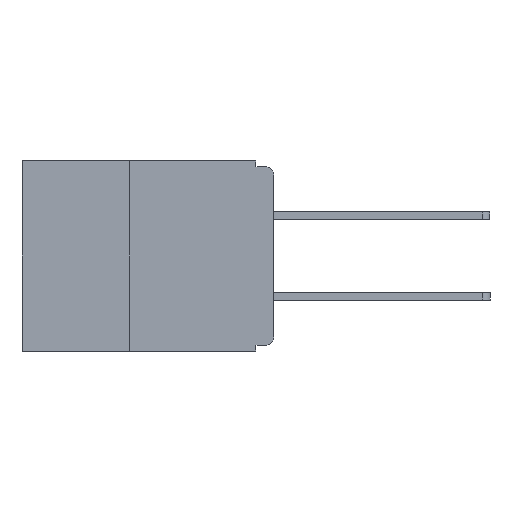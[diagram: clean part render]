
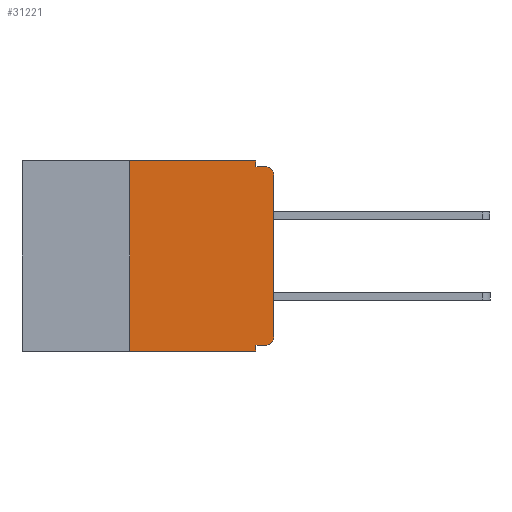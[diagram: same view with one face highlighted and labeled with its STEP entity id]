
A CAD part, left-side view. The second image highlights one B-rep face of the part: STEP entity #31221.
In plain terms, the highlighted planar face has unit normal (-1, 0, 0).
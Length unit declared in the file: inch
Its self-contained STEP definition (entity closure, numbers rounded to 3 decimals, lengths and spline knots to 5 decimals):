
#661 = VECTOR ( 'NONE', #12780, 39.37008 ) ;
#692 = VERTEX_POINT ( 'NONE', #15216 ) ;
#861 = DIRECTION ( 'NONE',  ( 0., -1., 0. ) ) ;
#935 = VECTOR ( 'NONE', #861, 39.37008 ) ;
#1255 = DIRECTION ( 'NONE',  ( 1., 0., 0. ) ) ;
#2095 = EDGE_CURVE ( 'NONE', #27092, #12245, #24377, .T. ) ;
#3526 = ORIENTED_EDGE ( 'NONE', *, *, #18318, .F. ) ;
#3633 = CARTESIAN_POINT ( 'NONE',  ( 0., 0.031, -0.32 ) ) ;
#3645 = AXIS2_PLACEMENT_3D ( 'NONE', #30515, #15388, #32843 ) ;
#3947 = VECTOR ( 'NONE', #20908, 39.37008 ) ;
#4465 = EDGE_CURVE ( 'NONE', #5434, #27092, #16620, .T. ) ;
#4595 = CARTESIAN_POINT ( 'NONE',  ( 0., 0.015, -0.01 ) ) ;
#4870 = CARTESIAN_POINT ( 'NONE',  ( 0., 0., -0.025 ) ) ;
#5060 = LINE ( 'NONE', #9561, #24713 ) ;
#5434 = VERTEX_POINT ( 'NONE', #10609 ) ;
#5600 = CARTESIAN_POINT ( 'NONE',  ( 0., 0.015, -0.025 ) ) ;
#5918 = CARTESIAN_POINT ( 'NONE',  ( 0., 0., -0.32 ) ) ;
#6284 = ORIENTED_EDGE ( 'NONE', *, *, #7286, .T. ) ;
#6888 = EDGE_CURVE ( 'NONE', #30057, #20302, #17683, .T. ) ;
#7286 = EDGE_CURVE ( 'NONE', #16791, #15302, #32844, .T. ) ;
#7553 = CIRCLE ( 'NONE', #17757, 0.015 ) ;
#7909 = VECTOR ( 'NONE', #13725, 39.37008 ) ;
#8222 = DIRECTION ( 'NONE',  ( 0., 0., -1. ) ) ;
#8648 = ORIENTED_EDGE ( 'NONE', *, *, #17672, .F. ) ;
#8723 = LINE ( 'NONE', #5918, #7909 ) ;
#8930 = ORIENTED_EDGE ( 'NONE', *, *, #28791, .F. ) ;
#9232 = ORIENTED_EDGE ( 'NONE', *, *, #26837, .T. ) ;
#9561 = CARTESIAN_POINT ( 'NONE',  ( 0., 0.031, -0.33 ) ) ;
#10609 = CARTESIAN_POINT ( 'NONE',  ( 0., 0.031, 0. ) ) ;
#10789 = EDGE_LOOP ( 'NONE', ( #27962, #29104, #29452, #30525, #32851, #3526, #6284, #8648, #8930, #9232 ) ) ;
#12162 = DIRECTION ( 'NONE',  ( 0., 0., -1. ) ) ;
#12245 = VERTEX_POINT ( 'NONE', #4595 ) ;
#12780 = DIRECTION ( 'NONE',  ( 0., -1., 0. ) ) ;
#13725 = DIRECTION ( 'NONE',  ( 0., 1., 0. ) ) ;
#13828 = CARTESIAN_POINT ( 'NONE',  ( 0., 0.437, 0. ) ) ;
#13958 = LINE ( 'NONE', #13828, #935 ) ;
#14100 = PLANE ( 'NONE',  #14803 ) ;
#14543 = VERTEX_POINT ( 'NONE', #3633 ) ;
#14803 = AXIS2_PLACEMENT_3D ( 'NONE', #26886, #1255, #19388 ) ;
#15216 = CARTESIAN_POINT ( 'NONE',  ( 0., 0.25, 0. ) ) ;
#15302 = VERTEX_POINT ( 'NONE', #19739 ) ;
#15388 = DIRECTION ( 'NONE',  ( -1., 0., 0. ) ) ;
#15793 = VECTOR ( 'NONE', #28084, 39.37008 ) ;
#16620 = LINE ( 'NONE', #28332, #15793 ) ;
#16791 = VERTEX_POINT ( 'NONE', #25295 ) ;
#17085 = CARTESIAN_POINT ( 'NONE',  ( 0., 0., -0.305 ) ) ;
#17672 = EDGE_CURVE ( 'NONE', #14543, #15302, #5060, .T. ) ;
#17683 = LINE ( 'NONE', #25739, #3947 ) ;
#17757 = AXIS2_PLACEMENT_3D ( 'NONE', #5600, #23600, #8222 ) ;
#17824 = FACE_OUTER_BOUND ( 'NONE', #10789, .T. ) ;
#18318 = EDGE_CURVE ( 'NONE', #16791, #692, #19138, .T. ) ;
#19138 = LINE ( 'NONE', #24833, #32295 ) ;
#19388 = DIRECTION ( 'NONE',  ( 0., 0., -1. ) ) ;
#19739 = CARTESIAN_POINT ( 'NONE',  ( 0., 0.031, -0.33 ) ) ;
#20302 = VERTEX_POINT ( 'NONE', #4870 ) ;
#20908 = DIRECTION ( 'NONE',  ( 0., 0., 1. ) ) ;
#20918 = CIRCLE ( 'NONE', #3645, 0.015 ) ;
#21560 = CARTESIAN_POINT ( 'NONE',  ( 0., 0.031, -0.01 ) ) ;
#22231 = DIRECTION ( 'NONE',  ( 0., -1., 0. ) ) ;
#22416 = CARTESIAN_POINT ( 'NONE',  ( 0., 0., -0.01 ) ) ;
#22888 = VERTEX_POINT ( 'NONE', #28721 ) ;
#23600 = DIRECTION ( 'NONE',  ( -1., 0., 0. ) ) ;
#24377 = LINE ( 'NONE', #22416, #30187 ) ;
#24713 = VECTOR ( 'NONE', #12162, 39.37008 ) ;
#24833 = CARTESIAN_POINT ( 'NONE',  ( 0., 0.25, -0.33 ) ) ;
#25295 = CARTESIAN_POINT ( 'NONE',  ( 0., 0.25, -0.33 ) ) ;
#25739 = CARTESIAN_POINT ( 'NONE',  ( 0., 0., 0. ) ) ;
#26837 = EDGE_CURVE ( 'NONE', #22888, #30057, #20918, .T. ) ;
#26886 = CARTESIAN_POINT ( 'NONE',  ( 0., 0.437, 0. ) ) ;
#27092 = VERTEX_POINT ( 'NONE', #21560 ) ;
#27347 = DIRECTION ( 'NONE',  ( 0., 0., 1. ) ) ;
#27962 = ORIENTED_EDGE ( 'NONE', *, *, #6888, .T. ) ;
#28010 = CARTESIAN_POINT ( 'NONE',  ( 0., 0.437, -0.33 ) ) ;
#28084 = DIRECTION ( 'NONE',  ( 0., 0., -1. ) ) ;
#28137 = EDGE_CURVE ( 'NONE', #20302, #12245, #7553, .T. ) ;
#28332 = CARTESIAN_POINT ( 'NONE',  ( 0., 0.031, 0. ) ) ;
#28721 = CARTESIAN_POINT ( 'NONE',  ( 0., 0.015, -0.32 ) ) ;
#28791 = EDGE_CURVE ( 'NONE', #22888, #14543, #8723, .T. ) ;
#28835 = EDGE_CURVE ( 'NONE', #692, #5434, #13958, .T. ) ;
#29104 = ORIENTED_EDGE ( 'NONE', *, *, #28137, .T. ) ;
#29452 = ORIENTED_EDGE ( 'NONE', *, *, #2095, .F. ) ;
#30057 = VERTEX_POINT ( 'NONE', #17085 ) ;
#30187 = VECTOR ( 'NONE', #22231, 39.37008 ) ;
#30515 = CARTESIAN_POINT ( 'NONE',  ( 0., 0.015, -0.305 ) ) ;
#30525 = ORIENTED_EDGE ( 'NONE', *, *, #4465, .F. ) ;
#31221 = ADVANCED_FACE ( 'NONE', ( #17824 ), #14100, .F. ) ;
#32295 = VECTOR ( 'NONE', #27347, 39.37008 ) ;
#32843 = DIRECTION ( 'NONE',  ( 0., 0., -1. ) ) ;
#32844 = LINE ( 'NONE', #28010, #661 ) ;
#32851 = ORIENTED_EDGE ( 'NONE', *, *, #28835, .F. ) ;
